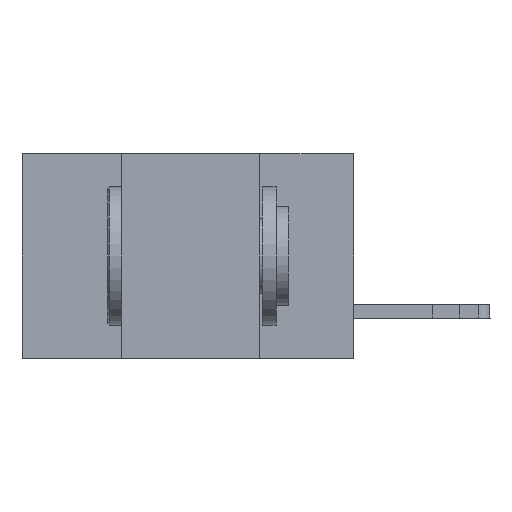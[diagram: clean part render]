
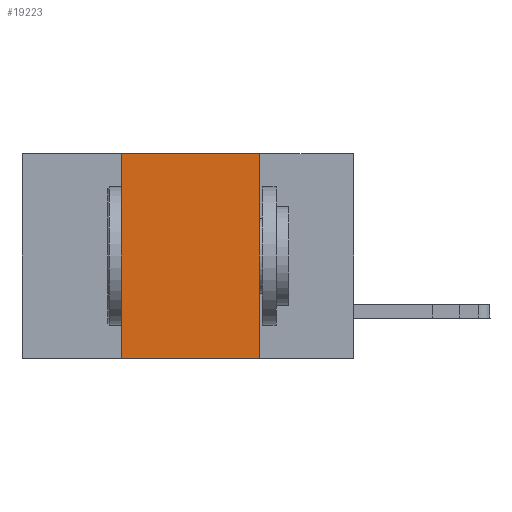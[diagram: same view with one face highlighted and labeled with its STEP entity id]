
A CAD part, left-side view. The second image highlights one B-rep face of the part: STEP entity #19223.
In plain terms, the highlighted planar face has unit normal (-1, 0, 0).
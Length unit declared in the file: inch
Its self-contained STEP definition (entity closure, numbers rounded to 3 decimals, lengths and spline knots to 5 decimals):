
#812 = CARTESIAN_POINT ( 'NONE',  ( 0., 0.17, 0. ) ) ;
#1811 = ORIENTED_EDGE ( 'NONE', *, *, #3306, .T. ) ;
#2053 = FACE_OUTER_BOUND ( 'NONE', #32294, .T. ) ;
#2109 = CARTESIAN_POINT ( 'NONE',  ( 0., 0.6, -0.37 ) ) ;
#3306 = EDGE_CURVE ( 'NONE', #23568, #16728, #34158, .T. ) ;
#4002 = CARTESIAN_POINT ( 'NONE',  ( 0., 0.17, -0.37 ) ) ;
#4225 = DIRECTION ( 'NONE',  ( 0., -1., 0. ) ) ;
#5945 = VECTOR ( 'NONE', #16899, 39.37008 ) ;
#6166 = CARTESIAN_POINT ( 'NONE',  ( 0., 0.42, 0. ) ) ;
#6585 = VECTOR ( 'NONE', #4225, 39.37008 ) ;
#7334 = LINE ( 'NONE', #9973, #18966 ) ;
#7507 = DIRECTION ( 'NONE',  ( 0., -1., 0. ) ) ;
#7769 = EDGE_CURVE ( 'NONE', #22496, #16728, #17619, .T. ) ;
#9421 = ORIENTED_EDGE ( 'NONE', *, *, #7769, .F. ) ;
#9973 = CARTESIAN_POINT ( 'NONE',  ( 0., 0.6, 0. ) ) ;
#12446 = DIRECTION ( 'NONE',  ( 1., 0., 0. ) ) ;
#14801 = VECTOR ( 'NONE', #17273, 39.37008 ) ;
#14926 = DIRECTION ( 'NONE',  ( 0., 0., -1. ) ) ;
#15099 = EDGE_CURVE ( 'NONE', #23568, #23168, #30307, .T. ) ;
#15148 = CARTESIAN_POINT ( 'NONE',  ( 0., 0.17, 0. ) ) ;
#16728 = VERTEX_POINT ( 'NONE', #4002 ) ;
#16846 = CARTESIAN_POINT ( 'NONE',  ( 0., 0.42, -0.37 ) ) ;
#16863 = EDGE_CURVE ( 'NONE', #23168, #22496, #7334, .T. ) ;
#16899 = DIRECTION ( 'NONE',  ( 0., 0., 1. ) ) ;
#17273 = DIRECTION ( 'NONE',  ( 0., 0., -1. ) ) ;
#17619 = LINE ( 'NONE', #15148, #14801 ) ;
#18966 = VECTOR ( 'NONE', #7507, 39.37008 ) ;
#19223 = ADVANCED_FACE ( 'NONE', ( #2053 ), #33423, .F. ) ;
#20215 = AXIS2_PLACEMENT_3D ( 'NONE', #28141, #12446, #14926 ) ;
#22496 = VERTEX_POINT ( 'NONE', #812 ) ;
#23168 = VERTEX_POINT ( 'NONE', #29461 ) ;
#23568 = VERTEX_POINT ( 'NONE', #16846 ) ;
#28141 = CARTESIAN_POINT ( 'NONE',  ( 0., 0.6, 0. ) ) ;
#29461 = CARTESIAN_POINT ( 'NONE',  ( 0., 0.42, 0. ) ) ;
#29475 = ORIENTED_EDGE ( 'NONE', *, *, #15099, .F. ) ;
#30307 = LINE ( 'NONE', #6166, #5945 ) ;
#32294 = EDGE_LOOP ( 'NONE', ( #9421, #33189, #29475, #1811 ) ) ;
#33189 = ORIENTED_EDGE ( 'NONE', *, *, #16863, .F. ) ;
#33423 = PLANE ( 'NONE',  #20215 ) ;
#34158 = LINE ( 'NONE', #2109, #6585 ) ;
